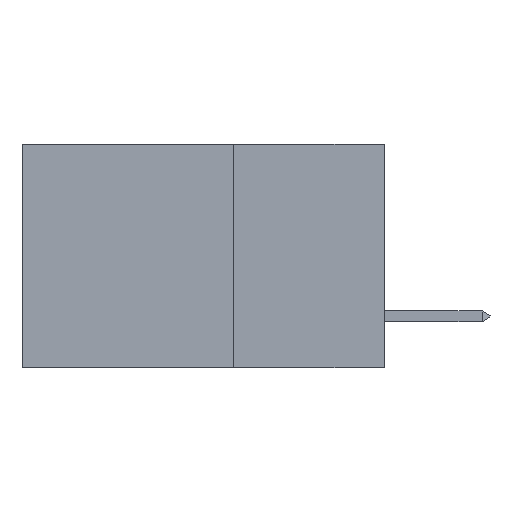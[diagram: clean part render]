
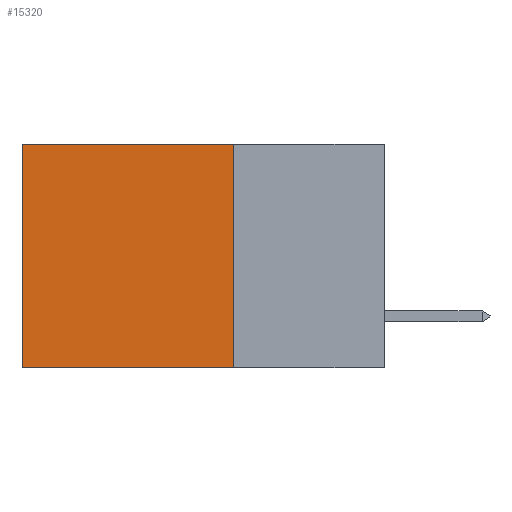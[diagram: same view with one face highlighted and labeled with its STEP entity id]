
A CAD part, left-side view. The second image highlights one B-rep face of the part: STEP entity #15320.
In plain terms, the highlighted planar face has unit normal (-1, 0, 0).
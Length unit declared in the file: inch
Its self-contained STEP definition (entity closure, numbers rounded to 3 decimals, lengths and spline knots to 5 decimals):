
#198 = DIRECTION ( 'NONE',  ( 0., 0., -1. ) ) ;
#561 = VERTEX_POINT ( 'NONE', #13984 ) ;
#586 = VERTEX_POINT ( 'NONE', #6907 ) ;
#1517 = DIRECTION ( 'NONE',  ( 0., 0., -1. ) ) ;
#1570 = EDGE_LOOP ( 'NONE', ( #6220, #4020, #15748, #10432 ) ) ;
#1695 = EDGE_CURVE ( 'NONE', #561, #586, #8388, .T. ) ;
#2542 = AXIS2_PLACEMENT_3D ( 'NONE', #13860, #6794, #1517 ) ;
#3065 = DIRECTION ( 'NONE',  ( 0., 0., -1. ) ) ;
#3965 = VECTOR ( 'NONE', #8874, 39.37008 ) ;
#4020 = ORIENTED_EDGE ( 'NONE', *, *, #5649, .F. ) ;
#4217 = VERTEX_POINT ( 'NONE', #12239 ) ;
#5192 = EDGE_CURVE ( 'NONE', #561, #4217, #5934, .T. ) ;
#5649 = EDGE_CURVE ( 'NONE', #4217, #12518, #6237, .T. ) ;
#5934 = LINE ( 'NONE', #8830, #14670 ) ;
#6220 = ORIENTED_EDGE ( 'NONE', *, *, #8687, .T. ) ;
#6237 = LINE ( 'NONE', #11690, #3965 ) ;
#6794 = DIRECTION ( 'NONE',  ( 1., 0., 0. ) ) ;
#6907 = CARTESIAN_POINT ( 'NONE',  ( 0.2875, 0.6, 0. ) ) ;
#6920 = VECTOR ( 'NONE', #3065, 39.37008 ) ;
#8297 = DIRECTION ( 'NONE',  ( 0., 1., 0. ) ) ;
#8388 = LINE ( 'NONE', #12480, #8513 ) ;
#8513 = VECTOR ( 'NONE', #8297, 39.37008 ) ;
#8687 = EDGE_CURVE ( 'NONE', #586, #12518, #16874, .T. ) ;
#8830 = CARTESIAN_POINT ( 'NONE',  ( 0.2875, 0.25, 0. ) ) ;
#8874 = DIRECTION ( 'NONE',  ( 0., 1., 0. ) ) ;
#9969 = CARTESIAN_POINT ( 'NONE',  ( 0.2875, 0.6, 0. ) ) ;
#10432 = ORIENTED_EDGE ( 'NONE', *, *, #1695, .T. ) ;
#11690 = CARTESIAN_POINT ( 'NONE',  ( 0.2875, 0.25, -0.37 ) ) ;
#12239 = CARTESIAN_POINT ( 'NONE',  ( 0.2875, 0.25, -0.37 ) ) ;
#12480 = CARTESIAN_POINT ( 'NONE',  ( 0.2875, 0.25, 0. ) ) ;
#12518 = VERTEX_POINT ( 'NONE', #16592 ) ;
#13860 = CARTESIAN_POINT ( 'NONE',  ( 0.2875, 0.25, 0. ) ) ;
#13955 = FACE_OUTER_BOUND ( 'NONE', #1570, .T. ) ;
#13984 = CARTESIAN_POINT ( 'NONE',  ( 0.2875, 0.25, 0. ) ) ;
#14670 = VECTOR ( 'NONE', #198, 39.37008 ) ;
#15039 = PLANE ( 'NONE',  #2542 ) ;
#15320 = ADVANCED_FACE ( 'NONE', ( #13955 ), #15039, .F. ) ;
#15748 = ORIENTED_EDGE ( 'NONE', *, *, #5192, .F. ) ;
#16592 = CARTESIAN_POINT ( 'NONE',  ( 0.2875, 0.6, -0.37 ) ) ;
#16874 = LINE ( 'NONE', #9969, #6920 ) ;
